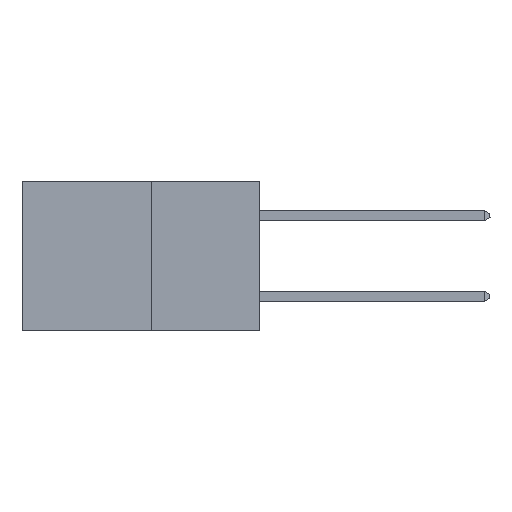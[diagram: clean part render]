
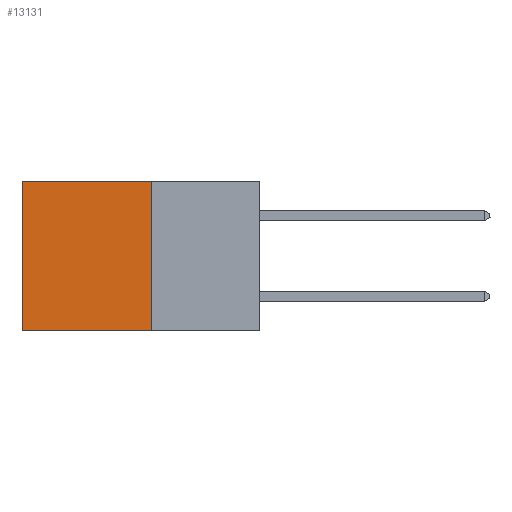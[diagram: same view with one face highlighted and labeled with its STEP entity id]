
A CAD part, left-side view. The second image highlights one B-rep face of the part: STEP entity #13131.
In plain terms, the highlighted planar face has unit normal (-1, 0, 0).
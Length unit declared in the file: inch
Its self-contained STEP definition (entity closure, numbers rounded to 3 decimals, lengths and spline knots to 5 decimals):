
#602 = CARTESIAN_POINT ( 'NONE',  ( 0.277, 0.27, -0.37 ) ) ;
#1146 = ORIENTED_EDGE ( 'NONE', *, *, #17424, .F. ) ;
#1169 = VERTEX_POINT ( 'NONE', #21088 ) ;
#1515 = ORIENTED_EDGE ( 'NONE', *, *, #2595, .F. ) ;
#2595 = EDGE_CURVE ( 'NONE', #14789, #3323, #17131, .T. ) ;
#3301 = ORIENTED_EDGE ( 'NONE', *, *, #11465, .T. ) ;
#3323 = VERTEX_POINT ( 'NONE', #21663 ) ;
#5641 = EDGE_CURVE ( 'NONE', #5988, #1169, #19116, .T. ) ;
#5793 = LINE ( 'NONE', #602, #19163 ) ;
#5988 = VERTEX_POINT ( 'NONE', #12971 ) ;
#7493 = LINE ( 'NONE', #7728, #10908 ) ;
#7663 = DIRECTION ( 'NONE',  ( 0., 0., -1. ) ) ;
#7728 = CARTESIAN_POINT ( 'NONE',  ( 0.277, 0.27, 0. ) ) ;
#7934 = CARTESIAN_POINT ( 'NONE',  ( 0.277, 0.27, -0.37 ) ) ;
#9995 = EDGE_LOOP ( 'NONE', ( #20443, #1146, #1515, #3301 ) ) ;
#10908 = VECTOR ( 'NONE', #14488, 39.37008 ) ;
#11465 = EDGE_CURVE ( 'NONE', #14789, #5988, #7493, .T. ) ;
#11529 = CARTESIAN_POINT ( 'NONE',  ( 0.277, 0.27, -0.37 ) ) ;
#11579 = PLANE ( 'NONE',  #17028 ) ;
#11850 = VECTOR ( 'NONE', #12502, 39.37008 ) ;
#12502 = DIRECTION ( 'NONE',  ( 0., 0., -1. ) ) ;
#12612 = DIRECTION ( 'NONE',  ( 0., 1., 0. ) ) ;
#12971 = CARTESIAN_POINT ( 'NONE',  ( 0.277, 0.59, 0. ) ) ;
#13010 = DIRECTION ( 'NONE',  ( 0., 0., -1. ) ) ;
#13079 = DIRECTION ( 'NONE',  ( 1., 0., 0. ) ) ;
#13131 = ADVANCED_FACE ( 'NONE', ( #15208 ), #11579, .F. ) ;
#14488 = DIRECTION ( 'NONE',  ( 0., 1., 0. ) ) ;
#14789 = VERTEX_POINT ( 'NONE', #17021 ) ;
#15208 = FACE_OUTER_BOUND ( 'NONE', #9995, .T. ) ;
#16603 = VECTOR ( 'NONE', #7663, 39.37008 ) ;
#17021 = CARTESIAN_POINT ( 'NONE',  ( 0.277, 0.27, 0. ) ) ;
#17028 = AXIS2_PLACEMENT_3D ( 'NONE', #11529, #13079, #13010 ) ;
#17131 = LINE ( 'NONE', #7934, #16603 ) ;
#17424 = EDGE_CURVE ( 'NONE', #3323, #1169, #5793, .T. ) ;
#19116 = LINE ( 'NONE', #20082, #11850 ) ;
#19163 = VECTOR ( 'NONE', #12612, 39.37008 ) ;
#20082 = CARTESIAN_POINT ( 'NONE',  ( 0.277, 0.59, -0.37 ) ) ;
#20443 = ORIENTED_EDGE ( 'NONE', *, *, #5641, .T. ) ;
#21088 = CARTESIAN_POINT ( 'NONE',  ( 0.277, 0.59, -0.37 ) ) ;
#21663 = CARTESIAN_POINT ( 'NONE',  ( 0.277, 0.27, -0.37 ) ) ;
